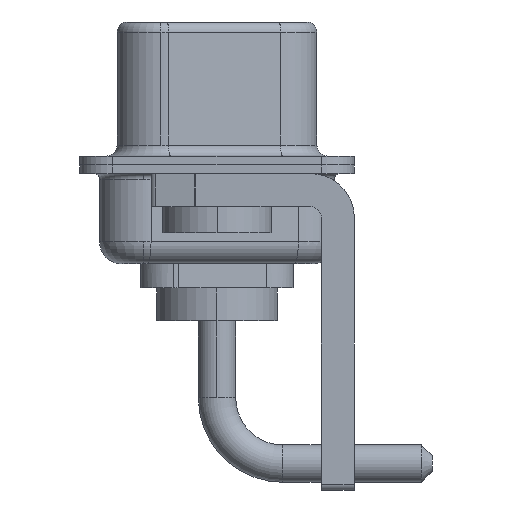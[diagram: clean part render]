
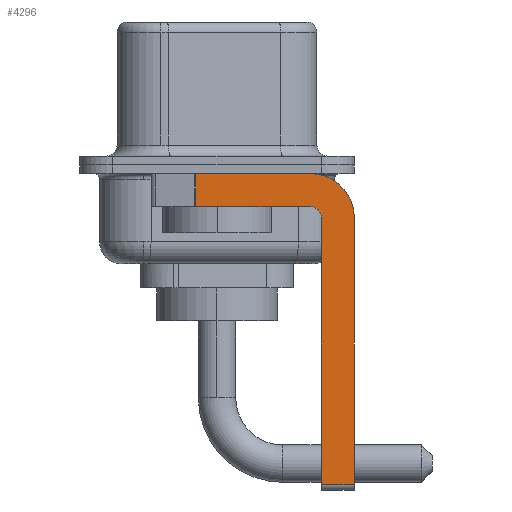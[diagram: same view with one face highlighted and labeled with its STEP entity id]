
A CAD part, left-side view. The second image highlights one B-rep face of the part: STEP entity #4296.
In plain terms, the highlighted planar face has unit normal (-1, 0, 0).
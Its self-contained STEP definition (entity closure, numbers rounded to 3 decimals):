
#49 = EDGE_CURVE ( 'NONE', #16499, #14574, #4471, .T. ) ;
#343 = EDGE_CURVE ( 'NONE', #14574, #15544, #2194, .T. ) ;
#1287 = DIRECTION ( 'NONE',  ( 1., 0., 0. ) ) ;
#1763 = CARTESIAN_POINT ( 'NONE',  ( -2.9, -4.25, -2.4 ) ) ;
#2194 = CIRCLE ( 'NONE', #7132, 0.5 ) ;
#2379 = EDGE_CURVE ( 'NONE', #4622, #13125, #4163, .T. ) ;
#2396 = CARTESIAN_POINT ( 'NONE',  ( -2.9, 0.978, -1.9 ) ) ;
#2413 = CARTESIAN_POINT ( 'NONE',  ( -2.9, -4.75, -14.55 ) ) ;
#2492 = DIRECTION ( 'NONE',  ( 0., 0., -1. ) ) ;
#3102 = DIRECTION ( 'NONE',  ( 0., 0., -1. ) ) ;
#3780 = EDGE_CURVE ( 'NONE', #10164, #14301, #7408, .T. ) ;
#4106 = PLANE ( 'NONE',  #11365 ) ;
#4163 = CIRCLE ( 'NONE', #7723, 2. ) ;
#4296 = ADVANCED_FACE ( 'NONE', ( #11936 ), #4106, .F. ) ;
#4471 = LINE ( 'NONE', #4727, #10974 ) ;
#4622 = VERTEX_POINT ( 'NONE', #11451 ) ;
#4674 = ORIENTED_EDGE ( 'NONE', *, *, #10553, .F. ) ;
#4727 = CARTESIAN_POINT ( 'NONE',  ( -2.9, -4.75, -14.8 ) ) ;
#5073 = ORIENTED_EDGE ( 'NONE', *, *, #3780, .T. ) ;
#5723 = DIRECTION ( 'NONE',  ( 0., -1., 0. ) ) ;
#5780 = VECTOR ( 'NONE', #5723, 1000. ) ;
#5884 = LINE ( 'NONE', #11132, #5780 ) ;
#6157 = LINE ( 'NONE', #7617, #15900 ) ;
#6540 = ORIENTED_EDGE ( 'NONE', *, *, #9113, .T. ) ;
#6741 = VECTOR ( 'NONE', #15326, 1000. ) ;
#6983 = ORIENTED_EDGE ( 'NONE', *, *, #343, .F. ) ;
#7132 = AXIS2_PLACEMENT_3D ( 'NONE', #1763, #14446, #13242 ) ;
#7242 = EDGE_CURVE ( 'NONE', #15544, #14301, #10871, .T. ) ;
#7408 = LINE ( 'NONE', #8068, #16873 ) ;
#7562 = CARTESIAN_POINT ( 'NONE',  ( -2.9, 3., -0.4 ) ) ;
#7617 = CARTESIAN_POINT ( 'NONE',  ( -2.9, -6.25, -2.4 ) ) ;
#7645 = CARTESIAN_POINT ( 'NONE',  ( -2.9, -4.25, -2.4 ) ) ;
#7723 = AXIS2_PLACEMENT_3D ( 'NONE', #7645, #1287, #2492 ) ;
#7955 = DIRECTION ( 'NONE',  ( 1., 0., 0. ) ) ;
#8068 = CARTESIAN_POINT ( 'NONE',  ( -2.9, 0.978, -1.9 ) ) ;
#8128 = DIRECTION ( 'NONE',  ( 0., 0., -1. ) ) ;
#8496 = DIRECTION ( 'NONE',  ( 0., 0., 1. ) ) ;
#9113 = EDGE_CURVE ( 'NONE', #16499, #12662, #5884, .T. ) ;
#9500 = CARTESIAN_POINT ( 'NONE',  ( -2.9, -4.25, -1.9 ) ) ;
#9513 = CARTESIAN_POINT ( 'NONE',  ( -2.9, -4.25, -2.4 ) ) ;
#9976 = LINE ( 'NONE', #7562, #6741 ) ;
#10164 = VERTEX_POINT ( 'NONE', #11974 ) ;
#10553 = EDGE_CURVE ( 'NONE', #10164, #4622, #9976, .T. ) ;
#10700 = ORIENTED_EDGE ( 'NONE', *, *, #49, .F. ) ;
#10717 = ORIENTED_EDGE ( 'NONE', *, *, #7242, .F. ) ;
#10792 = DIRECTION ( 'NONE',  ( 0., 1., 0. ) ) ;
#10871 = LINE ( 'NONE', #9500, #11977 ) ;
#10974 = VECTOR ( 'NONE', #8496, 1000. ) ;
#11132 = CARTESIAN_POINT ( 'NONE',  ( -2.9, -4.25, -14.55 ) ) ;
#11365 = AXIS2_PLACEMENT_3D ( 'NONE', #9513, #7955, #8128 ) ;
#11386 = CARTESIAN_POINT ( 'NONE',  ( -2.9, -6.25, -2.4 ) ) ;
#11411 = DIRECTION ( 'NONE',  ( 0., 0., -1. ) ) ;
#11451 = CARTESIAN_POINT ( 'NONE',  ( -2.9, -4.25, -0.4 ) ) ;
#11936 = FACE_OUTER_BOUND ( 'NONE', #15881, .T. ) ;
#11974 = CARTESIAN_POINT ( 'NONE',  ( -2.9, 0.978, -0.4 ) ) ;
#11977 = VECTOR ( 'NONE', #10792, 1000. ) ;
#12630 = CARTESIAN_POINT ( 'NONE',  ( -2.9, -4.75, -2.4 ) ) ;
#12662 = VERTEX_POINT ( 'NONE', #13769 ) ;
#13102 = ORIENTED_EDGE ( 'NONE', *, *, #14650, .F. ) ;
#13125 = VERTEX_POINT ( 'NONE', #11386 ) ;
#13242 = DIRECTION ( 'NONE',  ( 0., 0., 1. ) ) ;
#13260 = ORIENTED_EDGE ( 'NONE', *, *, #2379, .F. ) ;
#13769 = CARTESIAN_POINT ( 'NONE',  ( -2.9, -6.25, -14.55 ) ) ;
#14301 = VERTEX_POINT ( 'NONE', #2396 ) ;
#14446 = DIRECTION ( 'NONE',  ( -1., 0., 0. ) ) ;
#14574 = VERTEX_POINT ( 'NONE', #12630 ) ;
#14650 = EDGE_CURVE ( 'NONE', #13125, #12662, #6157, .T. ) ;
#15326 = DIRECTION ( 'NONE',  ( 0., -1., 0. ) ) ;
#15544 = VERTEX_POINT ( 'NONE', #16673 ) ;
#15881 = EDGE_LOOP ( 'NONE', ( #4674, #5073, #10717, #6983, #10700, #6540, #13102, #13260 ) ) ;
#15900 = VECTOR ( 'NONE', #11411, 1000. ) ;
#16499 = VERTEX_POINT ( 'NONE', #2413 ) ;
#16673 = CARTESIAN_POINT ( 'NONE',  ( -2.9, -4.25, -1.9 ) ) ;
#16873 = VECTOR ( 'NONE', #3102, 1000. ) ;
